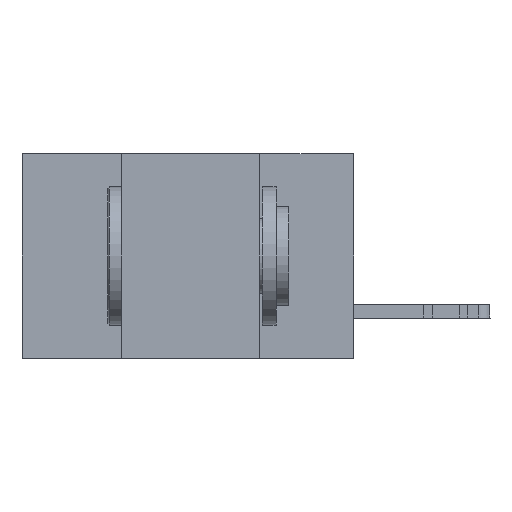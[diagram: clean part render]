
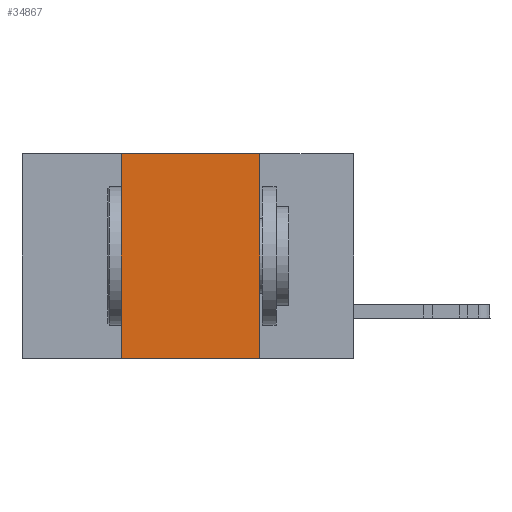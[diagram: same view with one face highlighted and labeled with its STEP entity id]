
A CAD part, left-side view. The second image highlights one B-rep face of the part: STEP entity #34867.
In plain terms, the highlighted planar face has unit normal (-1, 0, 0).
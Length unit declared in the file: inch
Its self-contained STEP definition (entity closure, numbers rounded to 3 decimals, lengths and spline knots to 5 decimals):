
#17 = VECTOR ( 'NONE', #5419, 39.37008 ) ;
#130 = VECTOR ( 'NONE', #2924, 39.37008 ) ;
#2924 = DIRECTION ( 'NONE',  ( 0., 0., -1. ) ) ;
#3481 = CARTESIAN_POINT ( 'NONE',  ( 0., 0.42, -0.37 ) ) ;
#4327 = PLANE ( 'NONE',  #24979 ) ;
#4754 = CARTESIAN_POINT ( 'NONE',  ( 0., 0.6, -0.37 ) ) ;
#5419 = DIRECTION ( 'NONE',  ( 0., -1., 0. ) ) ;
#10362 = LINE ( 'NONE', #23821, #12777 ) ;
#12507 = VERTEX_POINT ( 'NONE', #20309 ) ;
#12777 = VECTOR ( 'NONE', #37262, 39.37008 ) ;
#14165 = DIRECTION ( 'NONE',  ( 0., 0., -1. ) ) ;
#15112 = LINE ( 'NONE', #15968, #130 ) ;
#15968 = CARTESIAN_POINT ( 'NONE',  ( 0., 0.17, 0. ) ) ;
#17331 = EDGE_CURVE ( 'NONE', #34730, #12507, #10362, .T. ) ;
#19026 = EDGE_CURVE ( 'NONE', #34730, #38921, #22363, .T. ) ;
#20309 = CARTESIAN_POINT ( 'NONE',  ( 0., 0.42, 0. ) ) ;
#22363 = LINE ( 'NONE', #4754, #33894 ) ;
#23262 = CARTESIAN_POINT ( 'NONE',  ( 0., 0.17, 0. ) ) ;
#23821 = CARTESIAN_POINT ( 'NONE',  ( 0., 0.42, 0. ) ) ;
#24979 = AXIS2_PLACEMENT_3D ( 'NONE', #30395, #27409, #14165 ) ;
#25430 = ORIENTED_EDGE ( 'NONE', *, *, #38700, .F. ) ;
#26471 = EDGE_LOOP ( 'NONE', ( #25430, #38886, #33789, #30835 ) ) ;
#26984 = DIRECTION ( 'NONE',  ( 0., -1., 0. ) ) ;
#27029 = EDGE_CURVE ( 'NONE', #12507, #41995, #38733, .T. ) ;
#27409 = DIRECTION ( 'NONE',  ( 1., 0., 0. ) ) ;
#30395 = CARTESIAN_POINT ( 'NONE',  ( 0., 0.6, 0. ) ) ;
#30835 = ORIENTED_EDGE ( 'NONE', *, *, #19026, .T. ) ;
#33594 = FACE_OUTER_BOUND ( 'NONE', #26471, .T. ) ;
#33789 = ORIENTED_EDGE ( 'NONE', *, *, #17331, .F. ) ;
#33894 = VECTOR ( 'NONE', #26984, 39.37008 ) ;
#34730 = VERTEX_POINT ( 'NONE', #3481 ) ;
#34867 = ADVANCED_FACE ( 'NONE', ( #33594 ), #4327, .F. ) ;
#37262 = DIRECTION ( 'NONE',  ( 0., 0., 1. ) ) ;
#38700 = EDGE_CURVE ( 'NONE', #41995, #38921, #15112, .T. ) ;
#38733 = LINE ( 'NONE', #41514, #17 ) ;
#38886 = ORIENTED_EDGE ( 'NONE', *, *, #27029, .F. ) ;
#38921 = VERTEX_POINT ( 'NONE', #42023 ) ;
#41514 = CARTESIAN_POINT ( 'NONE',  ( 0., 0.6, 0. ) ) ;
#41995 = VERTEX_POINT ( 'NONE', #23262 ) ;
#42023 = CARTESIAN_POINT ( 'NONE',  ( 0., 0.17, -0.37 ) ) ;
